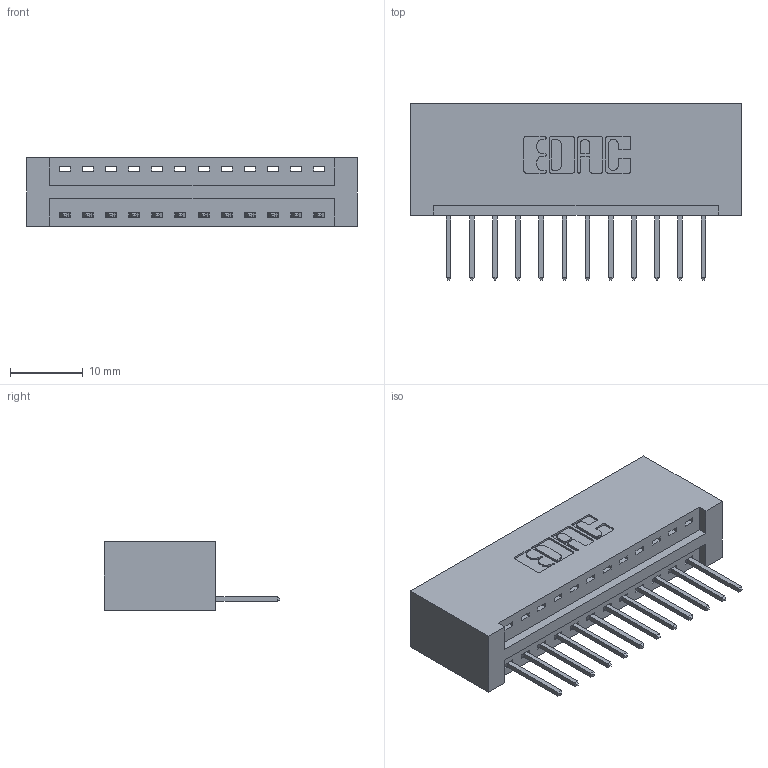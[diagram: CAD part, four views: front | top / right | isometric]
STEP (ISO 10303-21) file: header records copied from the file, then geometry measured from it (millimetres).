
FILE_DESCRIPTION (( 'STEP AP203' ), '1' );
FILE_NAME ('396-012-526-101.STEP', '2018-08-31T05:59:47', ( '' ), ( '' ), 'SwSTEP 2.0', 'SolidWorks 2016', '' );
FILE_SCHEMA (( 'CONFIG_CONTROL_DESIGN' ));
Length unit declared in the file: inch
Products named in the file (3): 396-012-526-101; 346 Part_No Mounting Lugs; 345-292-001_345-293-126
Assembly tree (13 placements, depth 2):
  396-012-526-101
    346 Part_No Mounting Lugs
    345-292-001_345-293-126  x12
Bounding box: 45.34 x 24.13 x 9.4 mm (x, y, z)
Volume: 4673.1 mm3; surface area: 5580.5 mm2
Topology: 13 solids, 13 shells, 810 faces, 2417 edges, 1594 vertices
Faces by surface type: plane 552, cylinder 258
Entity records: 11227 total; most frequent: CARTESIAN_POINT 1940, ORIENTED_EDGE 1886, DIRECTION 1743, EDGE_CURVE 943, VECTOR 771, LINE 771, VERTEX_POINT 626, AXIS2_PLACEMENT_3D 486
